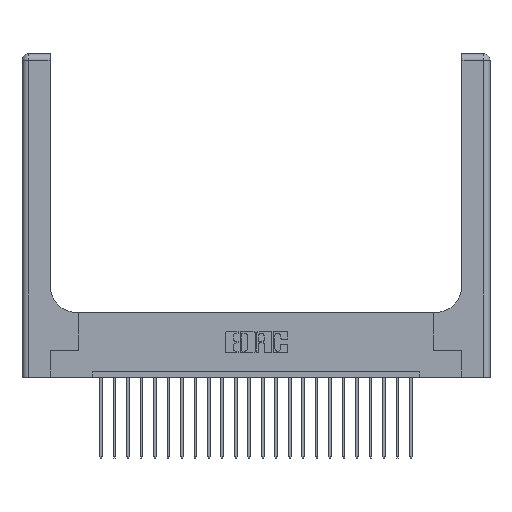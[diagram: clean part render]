
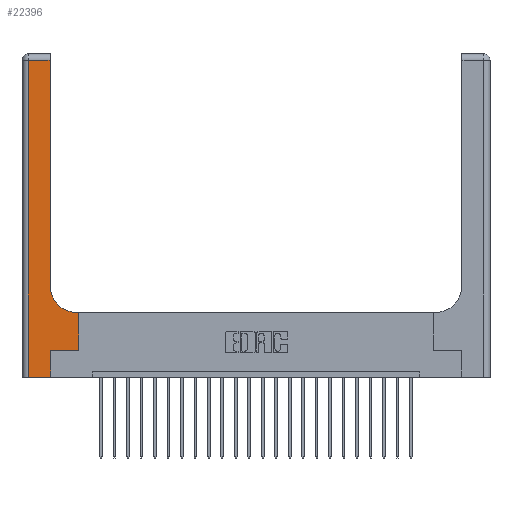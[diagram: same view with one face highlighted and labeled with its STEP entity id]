
A CAD part, top view. The second image highlights one B-rep face of the part: STEP entity #22396.
In plain terms, the highlighted planar face has unit normal (0, 0, 1).
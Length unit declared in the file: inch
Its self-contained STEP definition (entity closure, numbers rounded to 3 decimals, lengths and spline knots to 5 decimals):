
#681 = CARTESIAN_POINT ( 'NONE',  ( 0.528, 0.25, 0.37 ) ) ;
#789 = DIRECTION ( 'NONE',  ( 1., 0., 0. ) ) ;
#1438 = CARTESIAN_POINT ( 'NONE',  ( 0.265, 0., 0.37 ) ) ;
#1488 = CARTESIAN_POINT ( 'NONE',  ( 0.26, 0.85, 0.37 ) ) ;
#1497 = LINE ( 'NONE', #19423, #18082 ) ;
#2278 = CARTESIAN_POINT ( 'NONE',  ( 0.51, 0.6, 0.37 ) ) ;
#2455 = EDGE_CURVE ( 'NONE', #21584, #17097, #11776, .T. ) ;
#2900 = LINE ( 'NONE', #5950, #12620 ) ;
#3387 = DIRECTION ( 'NONE',  ( 0., 1., 0. ) ) ;
#3670 = DIRECTION ( 'NONE',  ( 1., 0., 0. ) ) ;
#4622 = AXIS2_PLACEMENT_3D ( 'NONE', #6658, #16948, #13207 ) ;
#4812 = EDGE_CURVE ( 'NONE', #17370, #21584, #22405, .T. ) ;
#5251 = ORIENTED_EDGE ( 'NONE', *, *, #7808, .T. ) ;
#5819 = VECTOR ( 'NONE', #3387, 39.37008 ) ;
#5950 = CARTESIAN_POINT ( 'NONE',  ( 0.26, 0.6, 0.37 ) ) ;
#6072 = CARTESIAN_POINT ( 'NONE',  ( 0., 2.94, 0.37 ) ) ;
#6105 = VECTOR ( 'NONE', #21306, 39.37008 ) ;
#6658 = CARTESIAN_POINT ( 'NONE',  ( 0., 3., 0.37 ) ) ;
#7145 = LINE ( 'NONE', #19209, #7429 ) ;
#7429 = VECTOR ( 'NONE', #15838, 39.37008 ) ;
#7498 = VERTEX_POINT ( 'NONE', #18798 ) ;
#7688 = CARTESIAN_POINT ( 'NONE',  ( 0., 0., 0.37 ) ) ;
#7796 = CARTESIAN_POINT ( 'NONE',  ( 0.06, 0., 0.37 ) ) ;
#7808 = EDGE_CURVE ( 'NONE', #12441, #15600, #2900, .T. ) ;
#7960 = VECTOR ( 'NONE', #11872, 39.37008 ) ;
#8013 = EDGE_CURVE ( 'NONE', #20948, #18763, #1497, .T. ) ;
#8232 = PLANE ( 'NONE',  #4622 ) ;
#8317 = CARTESIAN_POINT ( 'NONE',  ( 0.528, 0.25, 0.37 ) ) ;
#8717 = CARTESIAN_POINT ( 'NONE',  ( 0.265, 0.25, 0.37 ) ) ;
#9454 = ORIENTED_EDGE ( 'NONE', *, *, #8013, .T. ) ;
#9526 = ORIENTED_EDGE ( 'NONE', *, *, #11792, .T. ) ;
#9733 = FACE_OUTER_BOUND ( 'NONE', #22059, .T. ) ;
#9736 = CARTESIAN_POINT ( 'NONE',  ( 0.528, 0.6, 0.37 ) ) ;
#10317 = AXIS2_PLACEMENT_3D ( 'NONE', #16447, #21716, #789 ) ;
#11100 = ORIENTED_EDGE ( 'NONE', *, *, #2455, .T. ) ;
#11776 = LINE ( 'NONE', #7688, #22158 ) ;
#11792 = EDGE_CURVE ( 'NONE', #18763, #12441, #16104, .T. ) ;
#11872 = DIRECTION ( 'NONE',  ( 0., -1., 0. ) ) ;
#12317 = EDGE_CURVE ( 'NONE', #12500, #7498, #7145, .T. ) ;
#12405 = ORIENTED_EDGE ( 'NONE', *, *, #12417, .T. ) ;
#12417 = EDGE_CURVE ( 'NONE', #7498, #17370, #13349, .T. ) ;
#12441 = VERTEX_POINT ( 'NONE', #9736 ) ;
#12500 = VERTEX_POINT ( 'NONE', #1488 ) ;
#12620 = VECTOR ( 'NONE', #18086, 39.37008 ) ;
#12621 = ORIENTED_EDGE ( 'NONE', *, *, #13649, .T. ) ;
#13002 = ORIENTED_EDGE ( 'NONE', *, *, #19325, .T. ) ;
#13207 = DIRECTION ( 'NONE',  ( -1., 0., 0. ) ) ;
#13349 = LINE ( 'NONE', #6072, #17993 ) ;
#13649 = EDGE_CURVE ( 'NONE', #15600, #12500, #17137, .T. ) ;
#14219 = LINE ( 'NONE', #1438, #5819 ) ;
#14906 = CARTESIAN_POINT ( 'NONE',  ( 0.265, 0., 0.37 ) ) ;
#15600 = VERTEX_POINT ( 'NONE', #2278 ) ;
#15838 = DIRECTION ( 'NONE',  ( 0., 1., 0. ) ) ;
#16104 = LINE ( 'NONE', #681, #6105 ) ;
#16295 = ORIENTED_EDGE ( 'NONE', *, *, #12317, .T. ) ;
#16447 = CARTESIAN_POINT ( 'NONE',  ( 0.51, 0.85, 0.37 ) ) ;
#16948 = DIRECTION ( 'NONE',  ( 0., 0., -1. ) ) ;
#17097 = VERTEX_POINT ( 'NONE', #14906 ) ;
#17137 = CIRCLE ( 'NONE', #10317, 0.25 ) ;
#17208 = CARTESIAN_POINT ( 'NONE',  ( 0.06, 3., 0.37 ) ) ;
#17370 = VERTEX_POINT ( 'NONE', #17656 ) ;
#17656 = CARTESIAN_POINT ( 'NONE',  ( 0.06, 2.94, 0.37 ) ) ;
#17978 = ORIENTED_EDGE ( 'NONE', *, *, #4812, .T. ) ;
#17993 = VECTOR ( 'NONE', #18421, 39.37008 ) ;
#18082 = VECTOR ( 'NONE', #3670, 39.37008 ) ;
#18086 = DIRECTION ( 'NONE',  ( -1., 0., 0. ) ) ;
#18421 = DIRECTION ( 'NONE',  ( -1., 0., 0. ) ) ;
#18763 = VERTEX_POINT ( 'NONE', #8317 ) ;
#18798 = CARTESIAN_POINT ( 'NONE',  ( 0.26, 2.94, 0.37 ) ) ;
#19209 = CARTESIAN_POINT ( 'NONE',  ( 0.26, 3., 0.37 ) ) ;
#19325 = EDGE_CURVE ( 'NONE', #17097, #20948, #14219, .T. ) ;
#19423 = CARTESIAN_POINT ( 'NONE',  ( 0.265, 0.25, 0.37 ) ) ;
#19823 = DIRECTION ( 'NONE',  ( 1., 0., 0. ) ) ;
#20948 = VERTEX_POINT ( 'NONE', #8717 ) ;
#21306 = DIRECTION ( 'NONE',  ( 0., 1., 0. ) ) ;
#21584 = VERTEX_POINT ( 'NONE', #7796 ) ;
#21716 = DIRECTION ( 'NONE',  ( 0., 0., -1. ) ) ;
#22059 = EDGE_LOOP ( 'NONE', ( #16295, #12405, #17978, #11100, #13002, #9454, #9526, #5251, #12621 ) ) ;
#22158 = VECTOR ( 'NONE', #19823, 39.37008 ) ;
#22396 = ADVANCED_FACE ( 'NONE', ( #9733 ), #8232, .F. ) ;
#22405 = LINE ( 'NONE', #17208, #7960 ) ;
